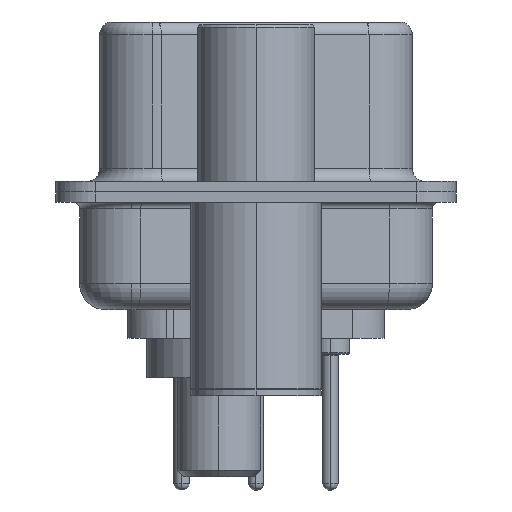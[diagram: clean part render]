
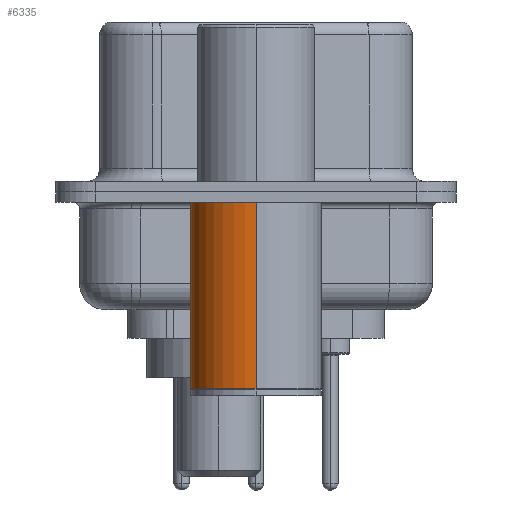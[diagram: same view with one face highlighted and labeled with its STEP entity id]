
A CAD part, left-side view. The second image highlights one B-rep face of the part: STEP entity #6335.
In plain terms, the highlighted cylindrical face has radius 2.5 mm (diameter 5 mm), a partial arc.
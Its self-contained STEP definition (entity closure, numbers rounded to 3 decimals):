
#364 = LINE ( 'NONE', #11209, #6944 ) ;
#507 = CARTESIAN_POINT ( 'NONE',  ( -2.5, 0., -0.4 ) ) ;
#1092 = VERTEX_POINT ( 'NONE', #27643 ) ;
#1935 = FACE_OUTER_BOUND ( 'NONE', #2361, .T. ) ;
#2361 = EDGE_LOOP ( 'NONE', ( #22050, #18468, #22575, #5903 ) ) ;
#2619 = VERTEX_POINT ( 'NONE', #11199 ) ;
#2959 = VERTEX_POINT ( 'NONE', #507 ) ;
#3241 = CARTESIAN_POINT ( 'NONE',  ( 0., 0., -0.4 ) ) ;
#4212 = DIRECTION ( 'NONE',  ( 0., 0., 1. ) ) ;
#4836 = DIRECTION ( 'NONE',  ( 0., 0., 1. ) ) ;
#5396 = DIRECTION ( 'NONE',  ( 1., 0., 0. ) ) ;
#5866 = VECTOR ( 'NONE', #4212, 1000. ) ;
#5903 = ORIENTED_EDGE ( 'NONE', *, *, #15765, .F. ) ;
#6041 = CIRCLE ( 'NONE', #11937, 2.5 ) ;
#6335 = ADVANCED_FACE ( 'NONE', ( #1935 ), #12781, .T. ) ;
#6944 = VECTOR ( 'NONE', #24191, 1000. ) ;
#7717 = DIRECTION ( 'NONE',  ( 0., 0., 1. ) ) ;
#7862 = DIRECTION ( 'NONE',  ( 1., 0., 0. ) ) ;
#10454 = EDGE_CURVE ( 'NONE', #1092, #2959, #23143, .T. ) ;
#10589 = CARTESIAN_POINT ( 'NONE',  ( -2.5, 0., 0.581 ) ) ;
#10830 = AXIS2_PLACEMENT_3D ( 'NONE', #3241, #18388, #5396 ) ;
#11199 = CARTESIAN_POINT ( 'NONE',  ( 2.5, 0., -7.525 ) ) ;
#11209 = CARTESIAN_POINT ( 'NONE',  ( 2.5, 0., 0.581 ) ) ;
#11815 = VERTEX_POINT ( 'NONE', #23910 ) ;
#11937 = AXIS2_PLACEMENT_3D ( 'NONE', #17793, #4836, #19988 ) ;
#12781 = CYLINDRICAL_SURFACE ( 'NONE', #27230, 2.5 ) ;
#13025 = EDGE_CURVE ( 'NONE', #2619, #1092, #6041, .T. ) ;
#13411 = EDGE_CURVE ( 'NONE', #11815, #2959, #25331, .T. ) ;
#15765 = EDGE_CURVE ( 'NONE', #2619, #11815, #364, .T. ) ;
#17793 = CARTESIAN_POINT ( 'NONE',  ( 0., 0., -7.525 ) ) ;
#18388 = DIRECTION ( 'NONE',  ( 0., 0., 1. ) ) ;
#18468 = ORIENTED_EDGE ( 'NONE', *, *, #10454, .T. ) ;
#19988 = DIRECTION ( 'NONE',  ( 1., 0., 0. ) ) ;
#22050 = ORIENTED_EDGE ( 'NONE', *, *, #13025, .T. ) ;
#22575 = ORIENTED_EDGE ( 'NONE', *, *, #13411, .F. ) ;
#23143 = LINE ( 'NONE', #10589, #5866 ) ;
#23448 = CARTESIAN_POINT ( 'NONE',  ( 0., 0., 0.581 ) ) ;
#23910 = CARTESIAN_POINT ( 'NONE',  ( 2.5, 0., -0.4 ) ) ;
#24191 = DIRECTION ( 'NONE',  ( 0., 0., 1. ) ) ;
#25331 = CIRCLE ( 'NONE', #10830, 2.5 ) ;
#27230 = AXIS2_PLACEMENT_3D ( 'NONE', #23448, #7717, #7862 ) ;
#27643 = CARTESIAN_POINT ( 'NONE',  ( -2.5, 0., -7.525 ) ) ;
